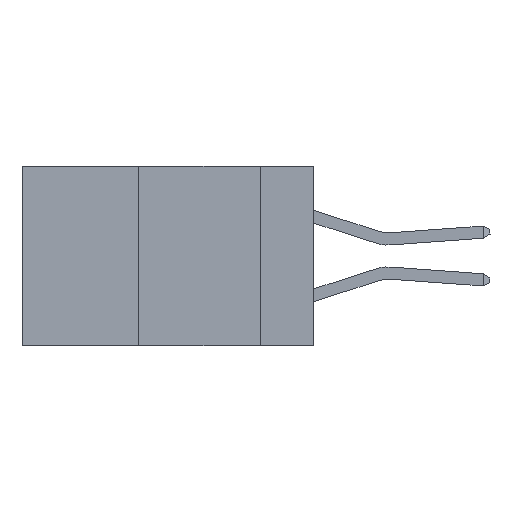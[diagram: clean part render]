
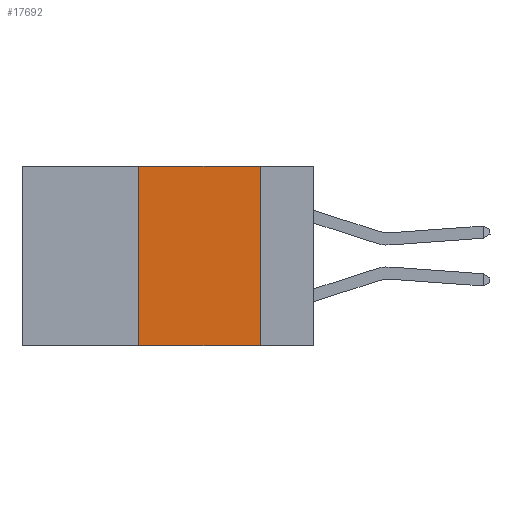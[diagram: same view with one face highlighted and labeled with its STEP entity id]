
A CAD part, left-side view. The second image highlights one B-rep face of the part: STEP entity #17692.
In plain terms, the highlighted planar face has unit normal (-1, 0, 0).
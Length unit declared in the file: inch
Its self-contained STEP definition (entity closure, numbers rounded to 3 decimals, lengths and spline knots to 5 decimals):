
#358 = CARTESIAN_POINT ( 'NONE',  ( 0., 0.11, 0. ) ) ;
#534 = CARTESIAN_POINT ( 'NONE',  ( 0., 0.36, 0. ) ) ;
#1340 = DIRECTION ( 'NONE',  ( 1., 0., 0. ) ) ;
#1773 = VECTOR ( 'NONE', #7173, 39.37008 ) ;
#2585 = VERTEX_POINT ( 'NONE', #8695 ) ;
#3110 = ORIENTED_EDGE ( 'NONE', *, *, #14166, .F. ) ;
#3143 = DIRECTION ( 'NONE',  ( 0., 0., -1. ) ) ;
#3488 = EDGE_LOOP ( 'NONE', ( #10591, #16263, #3110, #5425 ) ) ;
#3570 = EDGE_CURVE ( 'NONE', #15894, #2585, #7838, .T. ) ;
#3657 = LINE ( 'NONE', #358, #19686 ) ;
#3706 = VERTEX_POINT ( 'NONE', #9899 ) ;
#3977 = VECTOR ( 'NONE', #18912, 39.37008 ) ;
#5287 = CARTESIAN_POINT ( 'NONE',  ( 0., 0.6, 0. ) ) ;
#5425 = ORIENTED_EDGE ( 'NONE', *, *, #3570, .T. ) ;
#6653 = LINE ( 'NONE', #534, #1773 ) ;
#7060 = DIRECTION ( 'NONE',  ( 0., -1., 0. ) ) ;
#7173 = DIRECTION ( 'NONE',  ( 0., 0., 1. ) ) ;
#7838 = LINE ( 'NONE', #12265, #3977 ) ;
#8695 = CARTESIAN_POINT ( 'NONE',  ( 0., 0.11, -0.37 ) ) ;
#9899 = CARTESIAN_POINT ( 'NONE',  ( 0., 0.36, 0. ) ) ;
#10591 = ORIENTED_EDGE ( 'NONE', *, *, #17976, .F. ) ;
#10983 = LINE ( 'NONE', #5287, #16384 ) ;
#11476 = CARTESIAN_POINT ( 'NONE',  ( 0., 0.6, 0. ) ) ;
#12265 = CARTESIAN_POINT ( 'NONE',  ( 0., 0.6, -0.37 ) ) ;
#12586 = CARTESIAN_POINT ( 'NONE',  ( 0., 0.11, 0. ) ) ;
#13758 = AXIS2_PLACEMENT_3D ( 'NONE', #11476, #1340, #3143 ) ;
#14166 = EDGE_CURVE ( 'NONE', #15894, #3706, #6653, .T. ) ;
#14231 = CARTESIAN_POINT ( 'NONE',  ( 0., 0.36, -0.37 ) ) ;
#15762 = EDGE_CURVE ( 'NONE', #3706, #21384, #10983, .T. ) ;
#15894 = VERTEX_POINT ( 'NONE', #14231 ) ;
#16263 = ORIENTED_EDGE ( 'NONE', *, *, #15762, .F. ) ;
#16384 = VECTOR ( 'NONE', #7060, 39.37008 ) ;
#16989 = DIRECTION ( 'NONE',  ( 0., 0., -1. ) ) ;
#17692 = ADVANCED_FACE ( 'NONE', ( #20204 ), #19649, .F. ) ;
#17976 = EDGE_CURVE ( 'NONE', #21384, #2585, #3657, .T. ) ;
#18912 = DIRECTION ( 'NONE',  ( 0., -1., 0. ) ) ;
#19649 = PLANE ( 'NONE',  #13758 ) ;
#19686 = VECTOR ( 'NONE', #16989, 39.37008 ) ;
#20204 = FACE_OUTER_BOUND ( 'NONE', #3488, .T. ) ;
#21384 = VERTEX_POINT ( 'NONE', #12586 ) ;
